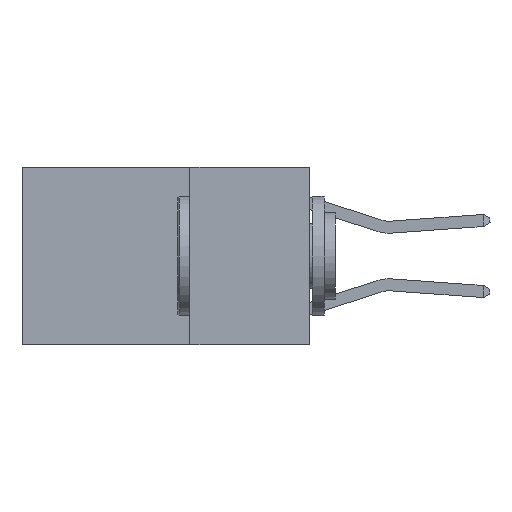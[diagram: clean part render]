
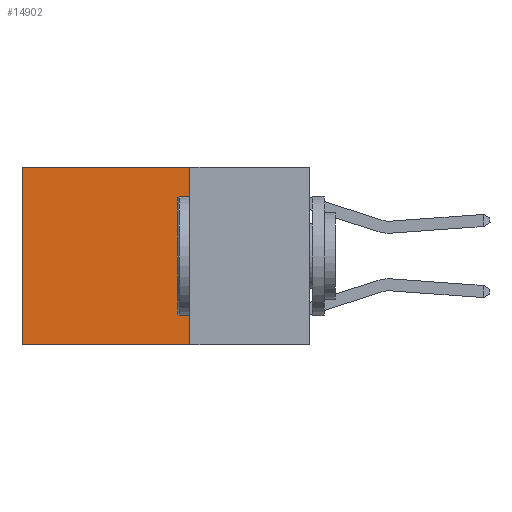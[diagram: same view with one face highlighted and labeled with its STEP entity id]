
A CAD part, left-side view. The second image highlights one B-rep face of the part: STEP entity #14902.
In plain terms, the highlighted planar face has unit normal (-1, 0, 0).
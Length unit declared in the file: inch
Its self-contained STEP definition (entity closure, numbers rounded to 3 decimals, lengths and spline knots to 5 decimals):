
#539 = DIRECTION ( 'NONE',  ( 0., 1., 0. ) ) ;
#1342 = FACE_OUTER_BOUND ( 'NONE', #11078, .T. ) ;
#1721 = CARTESIAN_POINT ( 'NONE',  ( 0.2625, 0.25, 0. ) ) ;
#1804 = EDGE_CURVE ( 'NONE', #14974, #11621, #18118, .T. ) ;
#2004 = ORIENTED_EDGE ( 'NONE', *, *, #1804, .F. ) ;
#2262 = EDGE_CURVE ( 'NONE', #10280, #17585, #18107, .T. ) ;
#2416 = CARTESIAN_POINT ( 'NONE',  ( 0.2625, 0.25, -0.37 ) ) ;
#2842 = CARTESIAN_POINT ( 'NONE',  ( 0.2625, 0.6, -0.37 ) ) ;
#6258 = DIRECTION ( 'NONE',  ( 0., 0., -1. ) ) ;
#6394 = CARTESIAN_POINT ( 'NONE',  ( 0.2625, 0.6, 0. ) ) ;
#6482 = VECTOR ( 'NONE', #539, 39.37008 ) ;
#6502 = VECTOR ( 'NONE', #8397, 39.37008 ) ;
#8112 = DIRECTION ( 'NONE',  ( 0., 0., -1. ) ) ;
#8130 = ORIENTED_EDGE ( 'NONE', *, *, #9471, .F. ) ;
#8144 = CARTESIAN_POINT ( 'NONE',  ( 0.2625, 0.25, -0.37 ) ) ;
#8397 = DIRECTION ( 'NONE',  ( 0., 1., 0. ) ) ;
#8561 = LINE ( 'NONE', #11226, #15919 ) ;
#9450 = LINE ( 'NONE', #16472, #16801 ) ;
#9471 = EDGE_CURVE ( 'NONE', #10280, #14974, #8561, .T. ) ;
#9834 = EDGE_CURVE ( 'NONE', #17585, #11621, #9450, .T. ) ;
#10280 = VERTEX_POINT ( 'NONE', #14489 ) ;
#11078 = EDGE_LOOP ( 'NONE', ( #15253, #2004, #8130, #17295 ) ) ;
#11226 = CARTESIAN_POINT ( 'NONE',  ( 0.2625, 0.25, 0. ) ) ;
#11621 = VERTEX_POINT ( 'NONE', #2842 ) ;
#11999 = AXIS2_PLACEMENT_3D ( 'NONE', #13966, #16889, #8112 ) ;
#12733 = DIRECTION ( 'NONE',  ( 0., 0., -1. ) ) ;
#13966 = CARTESIAN_POINT ( 'NONE',  ( 0.2625, 0.25, 0. ) ) ;
#14489 = CARTESIAN_POINT ( 'NONE',  ( 0.2625, 0.25, 0. ) ) ;
#14902 = ADVANCED_FACE ( 'NONE', ( #1342 ), #18255, .F. ) ;
#14974 = VERTEX_POINT ( 'NONE', #2416 ) ;
#15253 = ORIENTED_EDGE ( 'NONE', *, *, #9834, .T. ) ;
#15919 = VECTOR ( 'NONE', #12733, 39.37008 ) ;
#16472 = CARTESIAN_POINT ( 'NONE',  ( 0.2625, 0.6, 0. ) ) ;
#16801 = VECTOR ( 'NONE', #6258, 39.37008 ) ;
#16889 = DIRECTION ( 'NONE',  ( 1., 0., 0. ) ) ;
#17295 = ORIENTED_EDGE ( 'NONE', *, *, #2262, .T. ) ;
#17585 = VERTEX_POINT ( 'NONE', #6394 ) ;
#18107 = LINE ( 'NONE', #1721, #6482 ) ;
#18118 = LINE ( 'NONE', #8144, #6502 ) ;
#18255 = PLANE ( 'NONE',  #11999 ) ;
